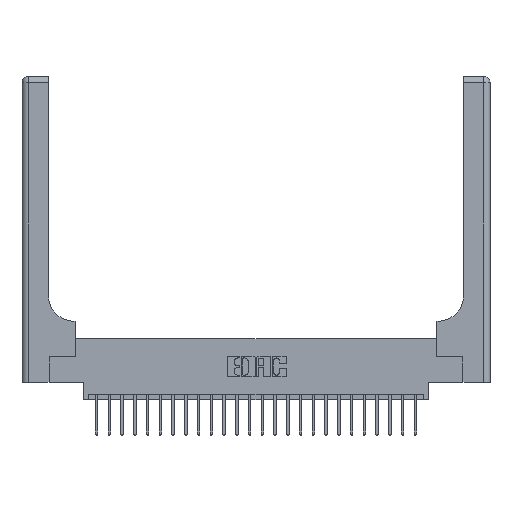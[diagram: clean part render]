
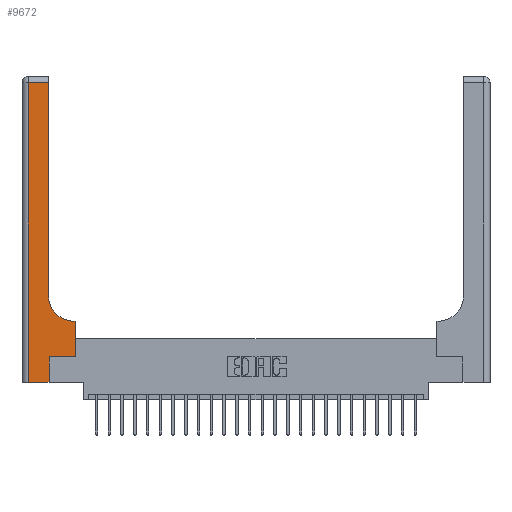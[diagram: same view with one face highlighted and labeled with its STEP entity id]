
A CAD part, top view. The second image highlights one B-rep face of the part: STEP entity #9672.
In plain terms, the highlighted planar face has unit normal (0, 0, 1).
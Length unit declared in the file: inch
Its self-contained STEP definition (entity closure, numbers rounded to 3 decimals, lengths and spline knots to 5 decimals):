
#32 = VECTOR ( 'NONE', #4795, 39.37008 ) ;
#216 = EDGE_LOOP ( 'NONE', ( #9941, #14457, #9041, #14545, #20912, #11928, #11670, #11988, #9649 ) ) ;
#452 = CARTESIAN_POINT ( 'NONE',  ( 0.26, 2.94, 0.37 ) ) ;
#1090 = DIRECTION ( 'NONE',  ( -1., 0., 0. ) ) ;
#1117 = CARTESIAN_POINT ( 'NONE',  ( 0.51, 0.85, 0.37 ) ) ;
#1590 = EDGE_CURVE ( 'NONE', #23266, #10346, #18931, .T. ) ;
#1628 = CARTESIAN_POINT ( 'NONE',  ( 0.26, 0.85, 0.37 ) ) ;
#2737 = VECTOR ( 'NONE', #10434, 39.37008 ) ;
#2745 = CARTESIAN_POINT ( 'NONE',  ( 0.265, 0., 0.37 ) ) ;
#2782 = LINE ( 'NONE', #6191, #4983 ) ;
#3246 = VERTEX_POINT ( 'NONE', #16111 ) ;
#3589 = EDGE_CURVE ( 'NONE', #10346, #20633, #4460, .T. ) ;
#4460 = LINE ( 'NONE', #14068, #24527 ) ;
#4758 = VECTOR ( 'NONE', #1090, 39.37008 ) ;
#4795 = DIRECTION ( 'NONE',  ( 0., 1., 0. ) ) ;
#4965 = CARTESIAN_POINT ( 'NONE',  ( 0.06, 2.94, 0.37 ) ) ;
#4983 = VECTOR ( 'NONE', #19562, 39.37008 ) ;
#6099 = LINE ( 'NONE', #7753, #21498 ) ;
#6191 = CARTESIAN_POINT ( 'NONE',  ( 0.265, 0.25, 0.37 ) ) ;
#7520 = CARTESIAN_POINT ( 'NONE',  ( 0., 3., 0.37 ) ) ;
#7642 = DIRECTION ( 'NONE',  ( -1., 0., 0. ) ) ;
#7753 = CARTESIAN_POINT ( 'NONE',  ( 0.06, 3., 0.37 ) ) ;
#9041 = ORIENTED_EDGE ( 'NONE', *, *, #17459, .T. ) ;
#9649 = ORIENTED_EDGE ( 'NONE', *, *, #1590, .T. ) ;
#9672 = ADVANCED_FACE ( 'NONE', ( #13343 ), #9786, .F. ) ;
#9786 = PLANE ( 'NONE',  #19160 ) ;
#9941 = ORIENTED_EDGE ( 'NONE', *, *, #3589, .T. ) ;
#10346 = VERTEX_POINT ( 'NONE', #1628 ) ;
#10434 = DIRECTION ( 'NONE',  ( -1., 0., 0. ) ) ;
#10550 = LINE ( 'NONE', #18375, #4758 ) ;
#10627 = VERTEX_POINT ( 'NONE', #12472 ) ;
#10862 = CARTESIAN_POINT ( 'NONE',  ( 0.528, 0.25, 0.37 ) ) ;
#11670 = ORIENTED_EDGE ( 'NONE', *, *, #11915, .T. ) ;
#11915 = EDGE_CURVE ( 'NONE', #10627, #19590, #24094, .T. ) ;
#11928 = ORIENTED_EDGE ( 'NONE', *, *, #16741, .T. ) ;
#11988 = ORIENTED_EDGE ( 'NONE', *, *, #22030, .T. ) ;
#12422 = CARTESIAN_POINT ( 'NONE',  ( 0.265, 0., 0.37 ) ) ;
#12472 = CARTESIAN_POINT ( 'NONE',  ( 0.528, 0.25, 0.37 ) ) ;
#13343 = FACE_OUTER_BOUND ( 'NONE', #216, .T. ) ;
#13487 = LINE ( 'NONE', #19381, #22840 ) ;
#13894 = CARTESIAN_POINT ( 'NONE',  ( 0.528, 0.6, 0.37 ) ) ;
#14068 = CARTESIAN_POINT ( 'NONE',  ( 0.26, 3., 0.37 ) ) ;
#14201 = VERTEX_POINT ( 'NONE', #15655 ) ;
#14457 = ORIENTED_EDGE ( 'NONE', *, *, #22063, .T. ) ;
#14498 = DIRECTION ( 'NONE',  ( 0., 1., 0. ) ) ;
#14545 = ORIENTED_EDGE ( 'NONE', *, *, #23107, .T. ) ;
#14747 = DIRECTION ( 'NONE',  ( 0., 0., -1. ) ) ;
#15098 = DIRECTION ( 'NONE',  ( 0., 0., -1. ) ) ;
#15456 = DIRECTION ( 'NONE',  ( 0., -1., 0. ) ) ;
#15487 = DIRECTION ( 'NONE',  ( 1., 0., 0. ) ) ;
#15655 = CARTESIAN_POINT ( 'NONE',  ( 0.265, 0.25, 0.37 ) ) ;
#16111 = CARTESIAN_POINT ( 'NONE',  ( 0.06, 0., 0.37 ) ) ;
#16242 = VERTEX_POINT ( 'NONE', #12422 ) ;
#16741 = EDGE_CURVE ( 'NONE', #14201, #10627, #2782, .T. ) ;
#17459 = EDGE_CURVE ( 'NONE', #22628, #3246, #6099, .T. ) ;
#17991 = LINE ( 'NONE', #21896, #2737 ) ;
#18375 = CARTESIAN_POINT ( 'NONE',  ( 0., 2.94, 0.37 ) ) ;
#18793 = VECTOR ( 'NONE', #14498, 39.37008 ) ;
#18931 = CIRCLE ( 'NONE', #24161, 0.25 ) ;
#19160 = AXIS2_PLACEMENT_3D ( 'NONE', #7520, #15098, #7642 ) ;
#19381 = CARTESIAN_POINT ( 'NONE',  ( 0., 0., 0.37 ) ) ;
#19562 = DIRECTION ( 'NONE',  ( 1., 0., 0. ) ) ;
#19590 = VERTEX_POINT ( 'NONE', #13894 ) ;
#19900 = LINE ( 'NONE', #2745, #18793 ) ;
#20134 = CARTESIAN_POINT ( 'NONE',  ( 0.51, 0.6, 0.37 ) ) ;
#20237 = EDGE_CURVE ( 'NONE', #16242, #14201, #19900, .T. ) ;
#20633 = VERTEX_POINT ( 'NONE', #452 ) ;
#20912 = ORIENTED_EDGE ( 'NONE', *, *, #20237, .T. ) ;
#21356 = DIRECTION ( 'NONE',  ( 0., 1., 0. ) ) ;
#21498 = VECTOR ( 'NONE', #15456, 39.37008 ) ;
#21896 = CARTESIAN_POINT ( 'NONE',  ( 0.26, 0.6, 0.37 ) ) ;
#22030 = EDGE_CURVE ( 'NONE', #19590, #23266, #17991, .T. ) ;
#22063 = EDGE_CURVE ( 'NONE', #20633, #22628, #10550, .T. ) ;
#22628 = VERTEX_POINT ( 'NONE', #4965 ) ;
#22840 = VECTOR ( 'NONE', #15487, 39.37008 ) ;
#23107 = EDGE_CURVE ( 'NONE', #3246, #16242, #13487, .T. ) ;
#23266 = VERTEX_POINT ( 'NONE', #20134 ) ;
#24094 = LINE ( 'NONE', #10862, #32 ) ;
#24161 = AXIS2_PLACEMENT_3D ( 'NONE', #1117, #14747, #24183 ) ;
#24183 = DIRECTION ( 'NONE',  ( 1., 0., 0. ) ) ;
#24527 = VECTOR ( 'NONE', #21356, 39.37008 ) ;
